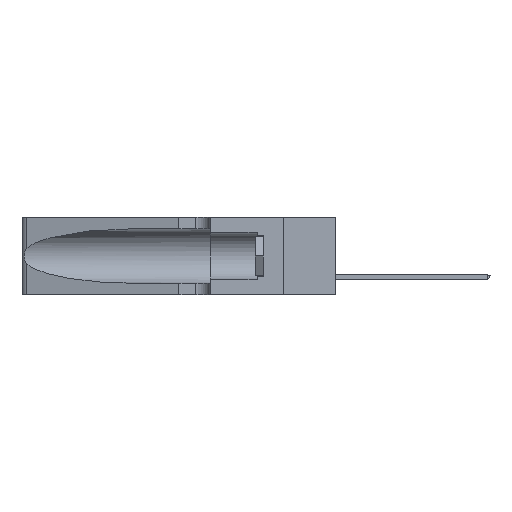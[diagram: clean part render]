
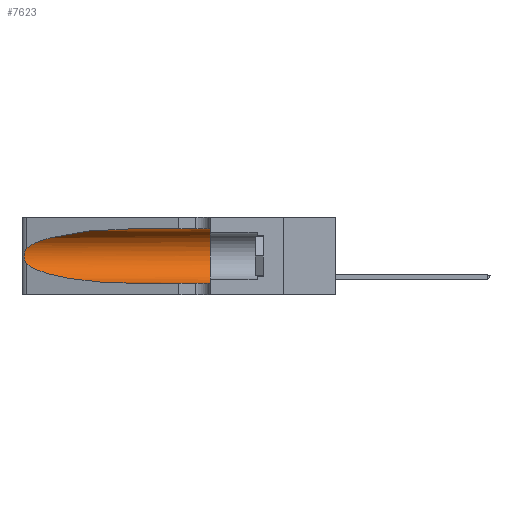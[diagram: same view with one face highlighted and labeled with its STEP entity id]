
A CAD part, left-side view. The second image highlights one B-rep face of the part: STEP entity #7623.
In plain terms, the highlighted cylindrical face has radius 3.308 mm (diameter 6.617 mm), a partial arc.
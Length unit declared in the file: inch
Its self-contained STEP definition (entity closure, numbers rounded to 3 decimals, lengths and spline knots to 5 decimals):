
#109 = VERTEX_POINT ( 'NONE', #2432 ) ;
#798 = ORIENTED_EDGE ( 'NONE', *, *, #37976, .T. ) ;
#1226 = CARTESIAN_POINT ( 'NONE',  ( 0.26075, 1.23896, 0.19203 ) ) ;
#2432 = CARTESIAN_POINT ( 'NONE',  ( 0.25487, 1.22718, 0.22369 ) ) ;
#2608 = EDGE_CURVE ( 'NONE', #26684, #35326, #21412, .T. ) ;
#2994 = DIRECTION ( 'NONE',  ( 0., -1., 0. ) ) ;
#3717 = EDGE_CURVE ( 'NONE', #35326, #10240, #26456, .T. ) ;
#3867 = CARTESIAN_POINT ( 'NONE',  ( 0.25639, 1.23184, 0.21858 ) ) ;
#6347 = DIRECTION ( 'NONE',  ( 0., 0., -1. ) ) ;
#6506 = LINE ( 'NONE', #19465, #43317 ) ;
#7623 = ADVANCED_FACE ( 'NONE', ( #14127 ), #10988, .F. ) ;
#8395 = ORIENTED_EDGE ( 'NONE', *, *, #18546, .F. ) ;
#9048 = DIRECTION ( 'NONE',  ( 0., -1., 0. ) ) ;
#10240 = VERTEX_POINT ( 'NONE', #33981 ) ;
#10590 =( BOUNDED_CURVE ( )  B_SPLINE_CURVE ( 3, ( #15065, #18626, #25709, #42027 ),
 .UNSPECIFIED., .F., .F. ) 
 B_SPLINE_CURVE_WITH_KNOTS ( ( 4, 4 ),
 ( 1.5708, 2.84003 ),
 .UNSPECIFIED. ) 
 CURVE ( )  GEOMETRIC_REPRESENTATION_ITEM ( )  RATIONAL_B_SPLINE_CURVE ( ( 1., 0.87, 0.87, 1. ) ) 
 REPRESENTATION_ITEM ( '' )  );
#10988 = CYLINDRICAL_SURFACE ( 'NONE', #33613, 0.13025 ) ;
#12167 = ORIENTED_EDGE ( 'NONE', *, *, #3717, .T. ) ;
#13496 = CARTESIAN_POINT ( 'NONE',  ( 0.26018, 1.23835, 0.19895 ) ) ;
#13894 = CARTESIAN_POINT ( 'NONE',  ( 0.25854, 1.2359, 0.20912 ) ) ;
#14127 = FACE_OUTER_BOUND ( 'NONE', #20560, .T. ) ;
#14487 = CARTESIAN_POINT ( 'NONE',  ( 0.25789, 1.23486, 0.15765 ) ) ;
#14665 = CARTESIAN_POINT ( 'NONE',  ( 0.1305, 1.61858, 0.05475 ) ) ;
#15065 = CARTESIAN_POINT ( 'NONE',  ( 0.1305, 0.72297, 0.31525 ) ) ;
#15092 = VERTEX_POINT ( 'NONE', #41744 ) ;
#16435 = VECTOR ( 'NONE', #31452, 39.37008 ) ;
#16975 = EDGE_CURVE ( 'NONE', #15092, #10240, #23426, .T. ) ;
#17788 = CARTESIAN_POINT ( 'NONE',  ( 0.18966, 0.96281, 0.05475 ) ) ;
#18546 = EDGE_CURVE ( 'NONE', #35255, #15092, #6506, .T. ) ;
#18626 = CARTESIAN_POINT ( 'NONE',  ( 0.18966, 0.96281, 0.31525 ) ) ;
#19465 = CARTESIAN_POINT ( 'NONE',  ( 0.1305, 1.61858, 0.31525 ) ) ;
#20560 = EDGE_LOOP ( 'NONE', ( #28986, #798, #26273, #12167, #36743, #8395 ) ) ;
#20962 = CARTESIAN_POINT ( 'NONE',  ( 0.25555, 1.22993, 0.14849 ) ) ;
#21412 =( BOUNDED_CURVE ( )  B_SPLINE_CURVE ( 3, ( #35124, #24382, #17788, #28374 ),
 .UNSPECIFIED., .F., .F. ) 
 B_SPLINE_CURVE_WITH_KNOTS ( ( 4, 4 ),
 ( 3.44316, 4.71239 ),
 .UNSPECIFIED. ) 
 CURVE ( )  GEOMETRIC_REPRESENTATION_ITEM ( )  RATIONAL_B_SPLINE_CURVE ( ( 1., 0.87, 0.87, 1. ) ) 
 REPRESENTATION_ITEM ( '' )  );
#21739 = DIRECTION ( 'NONE',  ( 0., 0., 1. ) ) ;
#23426 = CIRCLE ( 'NONE', #39520, 0.13025 ) ;
#24382 = CARTESIAN_POINT ( 'NONE',  ( 0.2373, 1.15595, 0.08982 ) ) ;
#24504 = CARTESIAN_POINT ( 'NONE',  ( 0.26017, 1.23833, 0.17102 ) ) ;
#24651 = CARTESIAN_POINT ( 'NONE',  ( 0.26075, 1.23896, 0.178 ) ) ;
#25709 = CARTESIAN_POINT ( 'NONE',  ( 0.2373, 1.15595, 0.28018 ) ) ;
#26273 = ORIENTED_EDGE ( 'NONE', *, *, #2608, .T. ) ;
#26456 = LINE ( 'NONE', #14665, #16435 ) ;
#26684 = VERTEX_POINT ( 'NONE', #28661 ) ;
#28034 = CARTESIAN_POINT ( 'NONE',  ( 0.1305, 0.35, 0.185 ) ) ;
#28374 = CARTESIAN_POINT ( 'NONE',  ( 0.1305, 0.72297, 0.05475 ) ) ;
#28661 = CARTESIAN_POINT ( 'NONE',  ( 0.25487, 1.22718, 0.14631 ) ) ;
#28986 = ORIENTED_EDGE ( 'NONE', *, *, #36946, .T. ) ;
#29646 = CARTESIAN_POINT ( 'NONE',  ( 0.1305, 1.61858, 0.185 ) ) ;
#30127 = CARTESIAN_POINT ( 'NONE',  ( 0.1305, 0.72297, 0.05475 ) ) ;
#31452 = DIRECTION ( 'NONE',  ( 0., -1., 0. ) ) ;
#31869 = DIRECTION ( 'NONE',  ( 0., 1., 0. ) ) ;
#33613 = AXIS2_PLACEMENT_3D ( 'NONE', #29646, #2994, #6347 ) ;
#33933 = CARTESIAN_POINT ( 'NONE',  ( 0.25555, 1.22994, 0.2215 ) ) ;
#33981 = CARTESIAN_POINT ( 'NONE',  ( 0.1305, 0.35, 0.05475 ) ) ;
#34068 = CARTESIAN_POINT ( 'NONE',  ( 0.25787, 1.23484, 0.2124 ) ) ;
#34780 = CARTESIAN_POINT ( 'NONE',  ( 0.25487, 1.22718, 0.14631 ) ) ;
#34831 = B_SPLINE_CURVE_WITH_KNOTS ( 'NONE', 3,
 ( #37053, #33933, #3867, #34068, #13894, #13496, #1226, #24651, #24504, #41583, #14487, #38035, #20962, #34780 ),
 .UNSPECIFIED., .F., .F.,
 ( 4, 2, 2, 2, 2, 2, 4 ),
 ( 0., 0.00027, 0.00053, 0.00107, 0.0016, 0.00187, 0.00214 ),
 .UNSPECIFIED. ) ;
#35124 = CARTESIAN_POINT ( 'NONE',  ( 0.25487, 1.22718, 0.14631 ) ) ;
#35255 = VERTEX_POINT ( 'NONE', #38276 ) ;
#35326 = VERTEX_POINT ( 'NONE', #30127 ) ;
#36743 = ORIENTED_EDGE ( 'NONE', *, *, #16975, .F. ) ;
#36946 = EDGE_CURVE ( 'NONE', #35255, #109, #10590, .T. ) ;
#37053 = CARTESIAN_POINT ( 'NONE',  ( 0.25487, 1.22718, 0.22369 ) ) ;
#37976 = EDGE_CURVE ( 'NONE', #109, #26684, #34831, .T. ) ;
#38035 = CARTESIAN_POINT ( 'NONE',  ( 0.25639, 1.23186, 0.15144 ) ) ;
#38276 = CARTESIAN_POINT ( 'NONE',  ( 0.1305, 0.72297, 0.31525 ) ) ;
#39520 = AXIS2_PLACEMENT_3D ( 'NONE', #28034, #31869, #21739 ) ;
#41583 = CARTESIAN_POINT ( 'NONE',  ( 0.25856, 1.23593, 0.16098 ) ) ;
#41744 = CARTESIAN_POINT ( 'NONE',  ( 0.1305, 0.35, 0.31525 ) ) ;
#42027 = CARTESIAN_POINT ( 'NONE',  ( 0.25487, 1.22718, 0.22369 ) ) ;
#43317 = VECTOR ( 'NONE', #9048, 39.37008 ) ;
